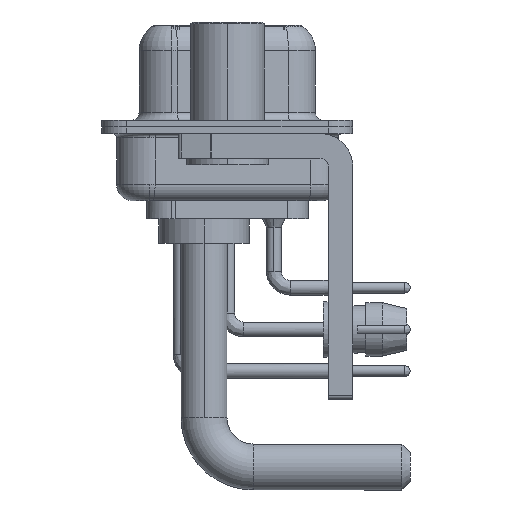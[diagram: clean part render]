
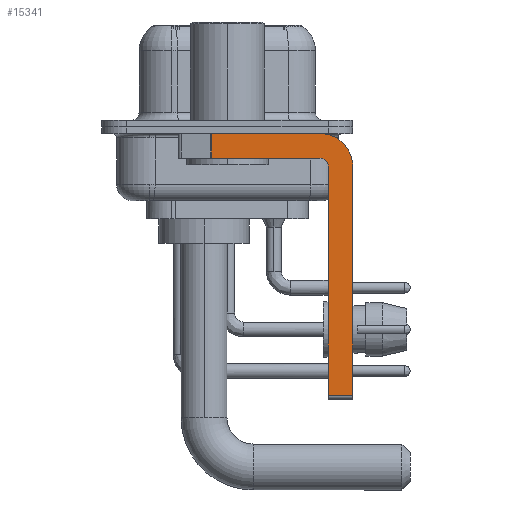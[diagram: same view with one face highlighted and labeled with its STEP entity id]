
A CAD part, left-side view. The second image highlights one B-rep face of the part: STEP entity #15341.
In plain terms, the highlighted planar face has unit normal (-1, 0, 0).
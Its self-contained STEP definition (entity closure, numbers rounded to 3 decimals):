
#525 = CARTESIAN_POINT ( 'NONE',  ( -2.9, -5.65, -1.9 ) ) ;
#4026 = VERTEX_POINT ( 'NONE', #9224 ) ;
#4354 = CARTESIAN_POINT ( 'NONE',  ( -2.9, 3., -0.4 ) ) ;
#5063 = DIRECTION ( 'NONE',  ( 0., 0., -1. ) ) ;
#5848 = DIRECTION ( 'NONE',  ( 0., 1., 0. ) ) ;
#6045 = EDGE_CURVE ( 'NONE', #4026, #27902, #11544, .T. ) ;
#6268 = ORIENTED_EDGE ( 'NONE', *, *, #7566, .F. ) ;
#6398 = VECTOR ( 'NONE', #23686, 1000. ) ;
#6447 = ORIENTED_EDGE ( 'NONE', *, *, #22839, .F. ) ;
#6845 = CARTESIAN_POINT ( 'NONE',  ( -2.9, -5.65, -0.4 ) ) ;
#7291 = LINE ( 'NONE', #35474, #15249 ) ;
#7473 = CARTESIAN_POINT ( 'NONE',  ( -2.9, 0.978, -1.9 ) ) ;
#7566 = EDGE_CURVE ( 'NONE', #16809, #20187, #14557, .T. ) ;
#7587 = LINE ( 'NONE', #13693, #34661 ) ;
#7752 = LINE ( 'NONE', #30208, #33125 ) ;
#8043 = PLANE ( 'NONE',  #14555 ) ;
#8210 = DIRECTION ( 'NONE',  ( 0., 0., 1. ) ) ;
#9014 = CARTESIAN_POINT ( 'NONE',  ( -2.9, -5.65, -1.9 ) ) ;
#9224 = CARTESIAN_POINT ( 'NONE',  ( -2.9, -6.15, -16.35 ) ) ;
#9394 = ORIENTED_EDGE ( 'NONE', *, *, #6045, .F. ) ;
#9715 = EDGE_LOOP ( 'NONE', ( #34963, #10347, #6268, #6447, #9394, #19085, #28324, #16282 ) ) ;
#10210 = DIRECTION ( 'NONE',  ( 0., 0., -1. ) ) ;
#10347 = ORIENTED_EDGE ( 'NONE', *, *, #33075, .T. ) ;
#10471 = CARTESIAN_POINT ( 'NONE',  ( -2.9, -5.65, -2.4 ) ) ;
#11187 = DIRECTION ( 'NONE',  ( 1., 0., 0. ) ) ;
#11544 = LINE ( 'NONE', #19905, #18622 ) ;
#12761 = CIRCLE ( 'NONE', #30536, 2. ) ;
#13143 = DIRECTION ( 'NONE',  ( 0., 0., -1. ) ) ;
#13693 = CARTESIAN_POINT ( 'NONE',  ( -2.9, 0.978, -1.9 ) ) ;
#14555 = AXIS2_PLACEMENT_3D ( 'NONE', #10471, #11187, #5063 ) ;
#14557 = LINE ( 'NONE', #9014, #33278 ) ;
#15249 = VECTOR ( 'NONE', #16373, 1000. ) ;
#15341 = ADVANCED_FACE ( 'NONE', ( #30494 ), #8043, .F. ) ;
#16282 = ORIENTED_EDGE ( 'NONE', *, *, #29347, .F. ) ;
#16373 = DIRECTION ( 'NONE',  ( 0., -1., 0. ) ) ;
#16809 = VERTEX_POINT ( 'NONE', #525 ) ;
#17965 = EDGE_CURVE ( 'NONE', #4026, #19755, #7291, .T. ) ;
#18269 = DIRECTION ( 'NONE',  ( 0., 0., 1. ) ) ;
#18622 = VECTOR ( 'NONE', #8210, 1000. ) ;
#18628 = CARTESIAN_POINT ( 'NONE',  ( -2.9, -5.65, -2.4 ) ) ;
#19085 = ORIENTED_EDGE ( 'NONE', *, *, #17965, .T. ) ;
#19755 = VERTEX_POINT ( 'NONE', #21990 ) ;
#19905 = CARTESIAN_POINT ( 'NONE',  ( -2.9, -6.15, -16.6 ) ) ;
#20187 = VERTEX_POINT ( 'NONE', #7473 ) ;
#20876 = EDGE_CURVE ( 'NONE', #23391, #30207, #23870, .T. ) ;
#21477 = CARTESIAN_POINT ( 'NONE',  ( -2.9, -7.65, -2.4 ) ) ;
#21519 = DIRECTION ( 'NONE',  ( 0., 0., -1. ) ) ;
#21887 = EDGE_CURVE ( 'NONE', #25729, #19755, #7752, .T. ) ;
#21990 = CARTESIAN_POINT ( 'NONE',  ( -2.9, -7.65, -16.35 ) ) ;
#22839 = EDGE_CURVE ( 'NONE', #27902, #16809, #29079, .T. ) ;
#23096 = CARTESIAN_POINT ( 'NONE',  ( -2.9, -5.65, -2.4 ) ) ;
#23391 = VERTEX_POINT ( 'NONE', #36173 ) ;
#23686 = DIRECTION ( 'NONE',  ( 0., -1., 0. ) ) ;
#23870 = LINE ( 'NONE', #4354, #6398 ) ;
#24309 = DIRECTION ( 'NONE',  ( 1., 0., 0. ) ) ;
#25729 = VERTEX_POINT ( 'NONE', #21477 ) ;
#26723 = CARTESIAN_POINT ( 'NONE',  ( -2.9, -6.15, -2.4 ) ) ;
#27902 = VERTEX_POINT ( 'NONE', #26723 ) ;
#28324 = ORIENTED_EDGE ( 'NONE', *, *, #21887, .F. ) ;
#29079 = CIRCLE ( 'NONE', #33195, 0.5 ) ;
#29347 = EDGE_CURVE ( 'NONE', #30207, #25729, #12761, .T. ) ;
#30207 = VERTEX_POINT ( 'NONE', #6845 ) ;
#30208 = CARTESIAN_POINT ( 'NONE',  ( -2.9, -7.65, -2.4 ) ) ;
#30494 = FACE_OUTER_BOUND ( 'NONE', #9715, .T. ) ;
#30536 = AXIS2_PLACEMENT_3D ( 'NONE', #23096, #24309, #10210 ) ;
#33075 = EDGE_CURVE ( 'NONE', #23391, #20187, #7587, .T. ) ;
#33125 = VECTOR ( 'NONE', #13143, 1000. ) ;
#33195 = AXIS2_PLACEMENT_3D ( 'NONE', #18628, #35675, #18269 ) ;
#33278 = VECTOR ( 'NONE', #5848, 1000. ) ;
#34661 = VECTOR ( 'NONE', #21519, 1000. ) ;
#34963 = ORIENTED_EDGE ( 'NONE', *, *, #20876, .F. ) ;
#35474 = CARTESIAN_POINT ( 'NONE',  ( -2.9, -5.65, -16.35 ) ) ;
#35675 = DIRECTION ( 'NONE',  ( -1., 0., 0. ) ) ;
#36173 = CARTESIAN_POINT ( 'NONE',  ( -2.9, 0.978, -0.4 ) ) ;
